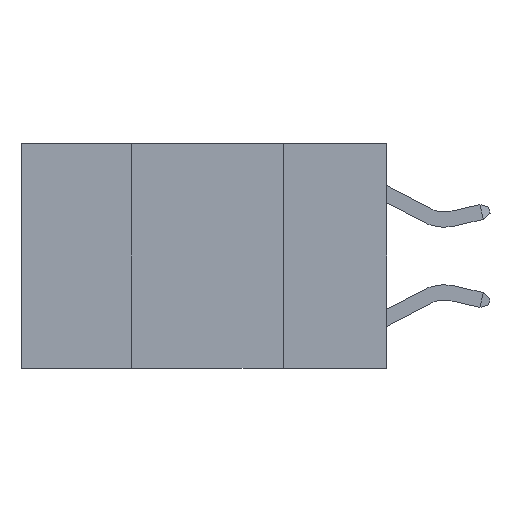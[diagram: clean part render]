
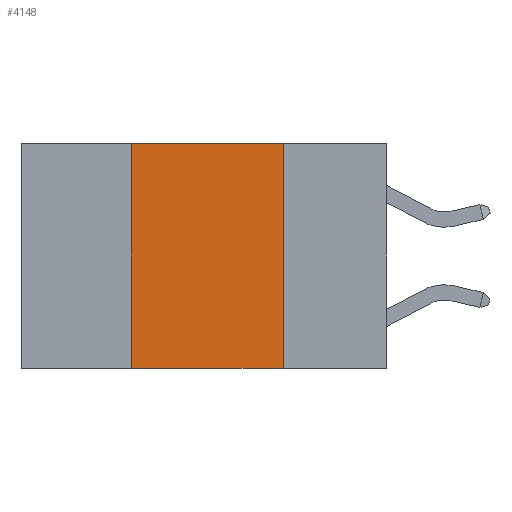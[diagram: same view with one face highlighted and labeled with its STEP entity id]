
A CAD part, left-side view. The second image highlights one B-rep face of the part: STEP entity #4148.
In plain terms, the highlighted planar face has unit normal (-1, 0, 0).
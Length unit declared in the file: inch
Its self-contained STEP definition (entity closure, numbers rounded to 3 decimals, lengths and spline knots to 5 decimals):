
#1012 = ORIENTED_EDGE ( 'NONE', *, *, #6722, .T. ) ;
#1842 = VECTOR ( 'NONE', #14085, 39.37008 ) ;
#2289 = LINE ( 'NONE', #4441, #1842 ) ;
#2521 = EDGE_CURVE ( 'NONE', #13435, #16951, #4010, .T. ) ;
#2617 = EDGE_CURVE ( 'NONE', #3118, #14602, #8912, .T. ) ;
#2903 = LINE ( 'NONE', #11014, #5380 ) ;
#2975 = EDGE_CURVE ( 'NONE', #14602, #13435, #2903, .T. ) ;
#3118 = VERTEX_POINT ( 'NONE', #14013 ) ;
#3878 = DIRECTION ( 'NONE',  ( 1., 0., 0. ) ) ;
#3961 = ORIENTED_EDGE ( 'NONE', *, *, #2521, .F. ) ;
#4010 = LINE ( 'NONE', #15347, #10580 ) ;
#4148 = ADVANCED_FACE ( 'NONE', ( #13500 ), #8145, .F. ) ;
#4441 = CARTESIAN_POINT ( 'NONE',  ( 0., 0.6, -0.37 ) ) ;
#4630 = CARTESIAN_POINT ( 'NONE',  ( 0., 0.42, 0. ) ) ;
#5380 = VECTOR ( 'NONE', #16297, 39.37008 ) ;
#6722 = EDGE_CURVE ( 'NONE', #3118, #16951, #2289, .T. ) ;
#6747 = CARTESIAN_POINT ( 'NONE',  ( 0., 0.6, 0. ) ) ;
#6906 = CARTESIAN_POINT ( 'NONE',  ( 0., 0.17, -0.37 ) ) ;
#7299 = DIRECTION ( 'NONE',  ( 0., 0., -1. ) ) ;
#8105 = CARTESIAN_POINT ( 'NONE',  ( 0., 0.17, 0. ) ) ;
#8145 = PLANE ( 'NONE',  #15589 ) ;
#8912 = LINE ( 'NONE', #4630, #15579 ) ;
#10131 = EDGE_LOOP ( 'NONE', ( #3961, #11401, #11843, #1012 ) ) ;
#10580 = VECTOR ( 'NONE', #7299, 39.37008 ) ;
#10717 = CARTESIAN_POINT ( 'NONE',  ( 0., 0.42, 0. ) ) ;
#11014 = CARTESIAN_POINT ( 'NONE',  ( 0., 0.6, 0. ) ) ;
#11401 = ORIENTED_EDGE ( 'NONE', *, *, #2975, .F. ) ;
#11843 = ORIENTED_EDGE ( 'NONE', *, *, #2617, .F. ) ;
#12940 = DIRECTION ( 'NONE',  ( 0., 0., 1. ) ) ;
#13435 = VERTEX_POINT ( 'NONE', #8105 ) ;
#13500 = FACE_OUTER_BOUND ( 'NONE', #10131, .T. ) ;
#13567 = DIRECTION ( 'NONE',  ( 0., 0., -1. ) ) ;
#14013 = CARTESIAN_POINT ( 'NONE',  ( 0., 0.42, -0.37 ) ) ;
#14085 = DIRECTION ( 'NONE',  ( 0., -1., 0. ) ) ;
#14602 = VERTEX_POINT ( 'NONE', #10717 ) ;
#15347 = CARTESIAN_POINT ( 'NONE',  ( 0., 0.17, 0. ) ) ;
#15579 = VECTOR ( 'NONE', #12940, 39.37008 ) ;
#15589 = AXIS2_PLACEMENT_3D ( 'NONE', #6747, #3878, #13567 ) ;
#16297 = DIRECTION ( 'NONE',  ( 0., -1., 0. ) ) ;
#16951 = VERTEX_POINT ( 'NONE', #6906 ) ;
